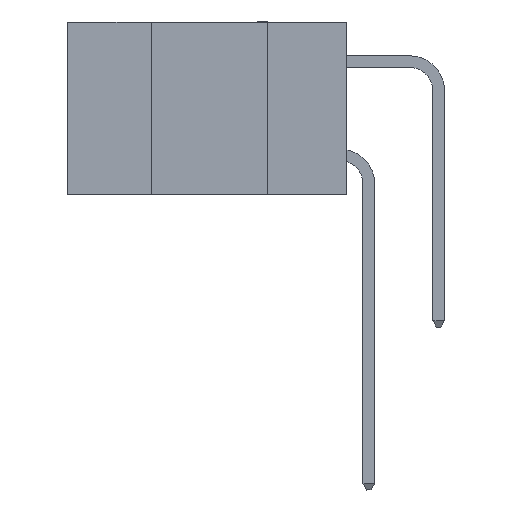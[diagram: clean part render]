
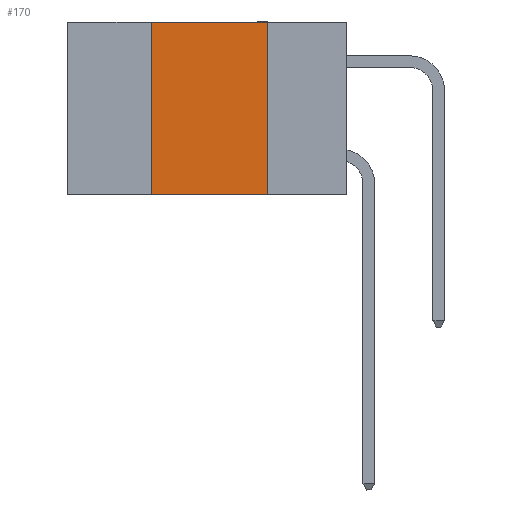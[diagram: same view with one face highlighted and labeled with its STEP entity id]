
A CAD part, left-side view. The second image highlights one B-rep face of the part: STEP entity #170.
In plain terms, the highlighted planar face has unit normal (-1, 0, 0).
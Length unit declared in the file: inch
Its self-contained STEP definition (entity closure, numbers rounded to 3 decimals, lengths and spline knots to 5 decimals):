
#170 = ADVANCED_FACE ( 'NONE', ( #7322 ), #32071, .F. ) ;
#597 = VECTOR ( 'NONE', #13654, 39.37008 ) ;
#838 = DIRECTION ( 'NONE',  ( 0., -1., 0. ) ) ;
#2208 = CARTESIAN_POINT ( 'NONE',  ( 0., 0.17, 0. ) ) ;
#2410 = CARTESIAN_POINT ( 'NONE',  ( 0., 0.42, -0.37 ) ) ;
#3599 = LINE ( 'NONE', #14140, #597 ) ;
#5245 = CARTESIAN_POINT ( 'NONE',  ( 0., 0.42, 0. ) ) ;
#5422 = DIRECTION ( 'NONE',  ( 0., 0., 1. ) ) ;
#6613 = CARTESIAN_POINT ( 'NONE',  ( 0., 0.17, 0. ) ) ;
#7322 = FACE_OUTER_BOUND ( 'NONE', #31353, .T. ) ;
#10048 = EDGE_CURVE ( 'NONE', #25768, #28757, #15807, .T. ) ;
#10156 = VECTOR ( 'NONE', #838, 39.37008 ) ;
#13472 = VECTOR ( 'NONE', #25146, 39.37008 ) ;
#13654 = DIRECTION ( 'NONE',  ( 0., -1., 0. ) ) ;
#14140 = CARTESIAN_POINT ( 'NONE',  ( 0., 0.6, 0. ) ) ;
#14758 = LINE ( 'NONE', #2208, #13472 ) ;
#15691 = EDGE_CURVE ( 'NONE', #28757, #25003, #3599, .T. ) ;
#15807 = LINE ( 'NONE', #5245, #26472 ) ;
#17399 = CARTESIAN_POINT ( 'NONE',  ( 0., 0.6, 0. ) ) ;
#17830 = LINE ( 'NONE', #28367, #10156 ) ;
#18044 = EDGE_CURVE ( 'NONE', #25768, #22627, #17830, .T. ) ;
#20387 = CARTESIAN_POINT ( 'NONE',  ( 0., 0.17, -0.37 ) ) ;
#21161 = ORIENTED_EDGE ( 'NONE', *, *, #15691, .F. ) ;
#22350 = DIRECTION ( 'NONE',  ( 0., 0., -1. ) ) ;
#22550 = EDGE_CURVE ( 'NONE', #25003, #22627, #14758, .T. ) ;
#22627 = VERTEX_POINT ( 'NONE', #20387 ) ;
#22665 = DIRECTION ( 'NONE',  ( 1., 0., 0. ) ) ;
#25003 = VERTEX_POINT ( 'NONE', #6613 ) ;
#25146 = DIRECTION ( 'NONE',  ( 0., 0., -1. ) ) ;
#25231 = ORIENTED_EDGE ( 'NONE', *, *, #18044, .T. ) ;
#25768 = VERTEX_POINT ( 'NONE', #2410 ) ;
#25912 = ORIENTED_EDGE ( 'NONE', *, *, #22550, .F. ) ;
#26472 = VECTOR ( 'NONE', #5422, 39.37008 ) ;
#27211 = AXIS2_PLACEMENT_3D ( 'NONE', #17399, #22665, #22350 ) ;
#28367 = CARTESIAN_POINT ( 'NONE',  ( 0., 0.6, -0.37 ) ) ;
#28757 = VERTEX_POINT ( 'NONE', #32081 ) ;
#28993 = ORIENTED_EDGE ( 'NONE', *, *, #10048, .F. ) ;
#31353 = EDGE_LOOP ( 'NONE', ( #25912, #21161, #28993, #25231 ) ) ;
#32071 = PLANE ( 'NONE',  #27211 ) ;
#32081 = CARTESIAN_POINT ( 'NONE',  ( 0., 0.42, 0. ) ) ;
